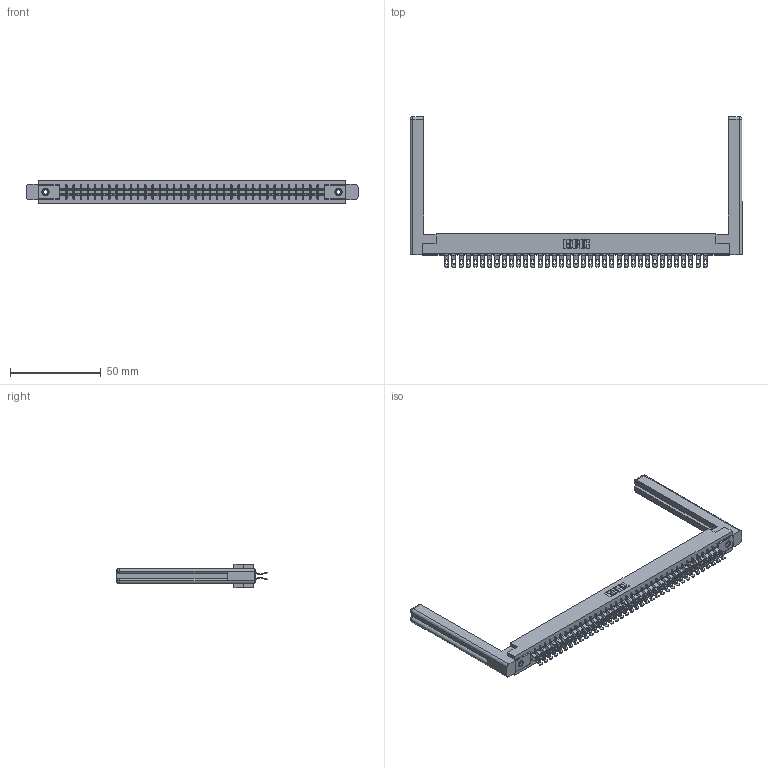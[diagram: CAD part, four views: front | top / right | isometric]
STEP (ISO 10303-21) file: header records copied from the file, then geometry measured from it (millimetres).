
FILE_DESCRIPTION (( 'STEP AP203' ), '1' );
FILE_NAME ('315-074-555-258.STEP', '2019-09-10T22:13:32', ( '' ), ( '' ), 'SwSTEP 2.0', 'SolidWorks 2016', '' );
FILE_SCHEMA (( 'CONFIG_CONTROL_DESIGN' ));
Length unit declared in the file: inch
Products named in the file (5): 305-290-001_555; 305 Part_.156 Dia; 315-074-555-258; 307-220-058; 345-250-001_345-250-001-102
Assembly tree (79 placements, depth 2):
  315-074-555-258
    305 Part_.156 Dia
    305-290-001_555  x74
    345-250-001_345-250-001-102  x2
    307-220-058  x2
Bounding box: 183.24 x 83.06 x 12.7 mm (x, y, z)
Volume: 26463.5 mm3; surface area: 30693.6 mm2
Topology: 79 solids, 79 shells, 5142 faces, 15285 edges, 9978 vertices
Faces by surface type: plane 2520, cylinder 2450, sphere 148, cone 12, torus 12
Entity records: 43927 total; most frequent: CARTESIAN_POINT 7302, ORIENTED_EDGE 7180, DIRECTION 7024, EDGE_CURVE 3590, VECTOR 2868, LINE 2868, VERTEX_POINT 2286, AXIS2_PLACEMENT_3D 2078
